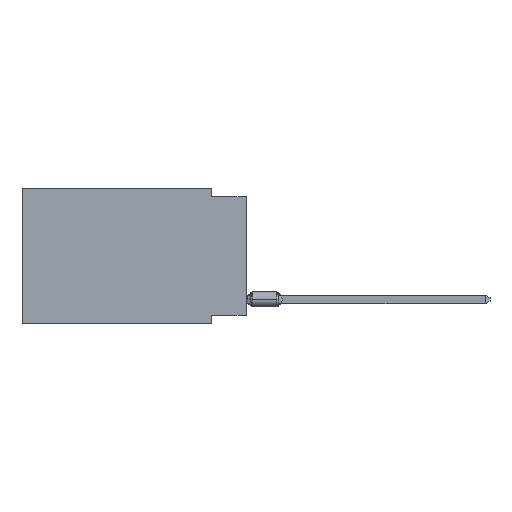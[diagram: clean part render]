
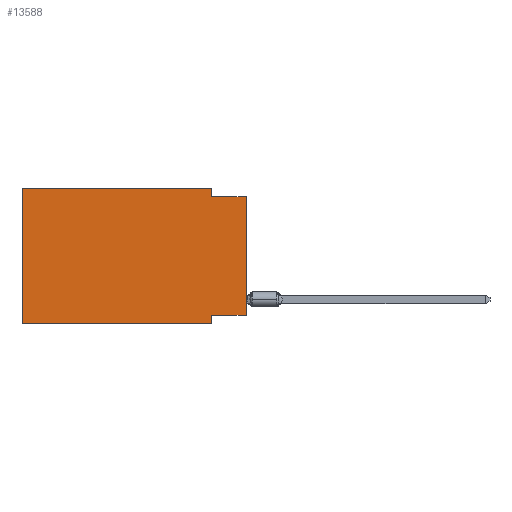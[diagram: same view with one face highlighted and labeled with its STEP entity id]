
A CAD part, left-side view. The second image highlights one B-rep face of the part: STEP entity #13588.
In plain terms, the highlighted planar face has unit normal (-1, 0, 0).
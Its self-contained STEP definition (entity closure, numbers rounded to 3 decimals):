
#491 = CARTESIAN_POINT ( 'NONE',  ( 0., 0., -0.635 ) ) ;
#715 = VECTOR ( 'NONE', #9395, 1000. ) ;
#747 = LINE ( 'NONE', #28103, #13635 ) ;
#829 = VECTOR ( 'NONE', #3011, 1000. ) ;
#838 = CARTESIAN_POINT ( 'NONE',  ( 0., 0., 0. ) ) ;
#1901 = CARTESIAN_POINT ( 'NONE',  ( 0., 0., -0.635 ) ) ;
#2153 = ORIENTED_EDGE ( 'NONE', *, *, #11407, .F. ) ;
#2697 = CARTESIAN_POINT ( 'NONE',  ( 0., 0., -9.271 ) ) ;
#2809 = DIRECTION ( 'NONE',  ( 0., 0., -1. ) ) ;
#3011 = DIRECTION ( 'NONE',  ( 0., -1., 0. ) ) ;
#3477 = CARTESIAN_POINT ( 'NONE',  ( 0., 2.54, 0. ) ) ;
#3535 = DIRECTION ( 'NONE',  ( 0., 0., -1. ) ) ;
#3694 = CARTESIAN_POINT ( 'NONE',  ( 0., 2.54, -9.271 ) ) ;
#3825 = DIRECTION ( 'NONE',  ( 0., -1., 0. ) ) ;
#4341 = PLANE ( 'NONE',  #7606 ) ;
#4815 = LINE ( 'NONE', #838, #26726 ) ;
#5224 = CARTESIAN_POINT ( 'NONE',  ( 0., 16.383, -9.906 ) ) ;
#6691 = VECTOR ( 'NONE', #2809, 1000. ) ;
#7606 = AXIS2_PLACEMENT_3D ( 'NONE', #20176, #18234, #27256 ) ;
#7804 = CARTESIAN_POINT ( 'NONE',  ( 0., 2.54, -9.906 ) ) ;
#8056 = LINE ( 'NONE', #13680, #715 ) ;
#8280 = ORIENTED_EDGE ( 'NONE', *, *, #9860, .F. ) ;
#9136 = CARTESIAN_POINT ( 'NONE',  ( 0., 16.383, 0. ) ) ;
#9204 = FACE_OUTER_BOUND ( 'NONE', #22629, .T. ) ;
#9395 = DIRECTION ( 'NONE',  ( 0., -1., 0. ) ) ;
#9860 = EDGE_CURVE ( 'NONE', #20263, #14290, #23783, .T. ) ;
#9905 = LINE ( 'NONE', #27944, #6691 ) ;
#9908 = CARTESIAN_POINT ( 'NONE',  ( 0., 2.54, -9.906 ) ) ;
#9975 = CARTESIAN_POINT ( 'NONE',  ( 0., 16.383, -9.906 ) ) ;
#10502 = VERTEX_POINT ( 'NONE', #491 ) ;
#11407 = EDGE_CURVE ( 'NONE', #17174, #20263, #18513, .T. ) ;
#11724 = DIRECTION ( 'NONE',  ( 0., 1., 0. ) ) ;
#12141 = VERTEX_POINT ( 'NONE', #9975 ) ;
#12301 = VECTOR ( 'NONE', #3825, 1000. ) ;
#12468 = LINE ( 'NONE', #5224, #829 ) ;
#12497 = VERTEX_POINT ( 'NONE', #21189 ) ;
#12509 = ORIENTED_EDGE ( 'NONE', *, *, #14121, .F. ) ;
#13028 = ORIENTED_EDGE ( 'NONE', *, *, #23773, .F. ) ;
#13084 = EDGE_CURVE ( 'NONE', #21373, #19651, #8056, .T. ) ;
#13588 = ADVANCED_FACE ( 'NONE', ( #9204 ), #4341, .F. ) ;
#13635 = VECTOR ( 'NONE', #20720, 1000. ) ;
#13680 = CARTESIAN_POINT ( 'NONE',  ( 0., 16.383, 0. ) ) ;
#14121 = EDGE_CURVE ( 'NONE', #19651, #12497, #9905, .T. ) ;
#14290 = VERTEX_POINT ( 'NONE', #7804 ) ;
#16359 = DIRECTION ( 'NONE',  ( 0., 0., 1. ) ) ;
#16847 = LINE ( 'NONE', #1901, #12301 ) ;
#17174 = VERTEX_POINT ( 'NONE', #18865 ) ;
#18234 = DIRECTION ( 'NONE',  ( 1., 0., 0. ) ) ;
#18513 = LINE ( 'NONE', #2697, #22850 ) ;
#18865 = CARTESIAN_POINT ( 'NONE',  ( 0., 0., -9.271 ) ) ;
#19382 = ORIENTED_EDGE ( 'NONE', *, *, #27280, .F. ) ;
#19486 = EDGE_CURVE ( 'NONE', #17174, #10502, #4815, .T. ) ;
#19651 = VERTEX_POINT ( 'NONE', #3477 ) ;
#20176 = CARTESIAN_POINT ( 'NONE',  ( 0., 16.383, 0. ) ) ;
#20263 = VERTEX_POINT ( 'NONE', #3694 ) ;
#20720 = DIRECTION ( 'NONE',  ( 0., 0., 1. ) ) ;
#21189 = CARTESIAN_POINT ( 'NONE',  ( 0., 2.54, -0.635 ) ) ;
#21373 = VERTEX_POINT ( 'NONE', #9136 ) ;
#22629 = EDGE_LOOP ( 'NONE', ( #25190, #19382, #12509, #23265, #13028, #29185, #8280, #2153 ) ) ;
#22850 = VECTOR ( 'NONE', #11724, 1000. ) ;
#23265 = ORIENTED_EDGE ( 'NONE', *, *, #13084, .F. ) ;
#23773 = EDGE_CURVE ( 'NONE', #12141, #21373, #747, .T. ) ;
#23783 = LINE ( 'NONE', #9908, #24255 ) ;
#24255 = VECTOR ( 'NONE', #3535, 1000. ) ;
#25190 = ORIENTED_EDGE ( 'NONE', *, *, #19486, .T. ) ;
#26726 = VECTOR ( 'NONE', #16359, 1000. ) ;
#27256 = DIRECTION ( 'NONE',  ( 0., 0., -1. ) ) ;
#27280 = EDGE_CURVE ( 'NONE', #12497, #10502, #16847, .T. ) ;
#27944 = CARTESIAN_POINT ( 'NONE',  ( 0., 2.54, 0. ) ) ;
#28103 = CARTESIAN_POINT ( 'NONE',  ( 0., 16.383, 0. ) ) ;
#29083 = EDGE_CURVE ( 'NONE', #12141, #14290, #12468, .T. ) ;
#29185 = ORIENTED_EDGE ( 'NONE', *, *, #29083, .T. ) ;
